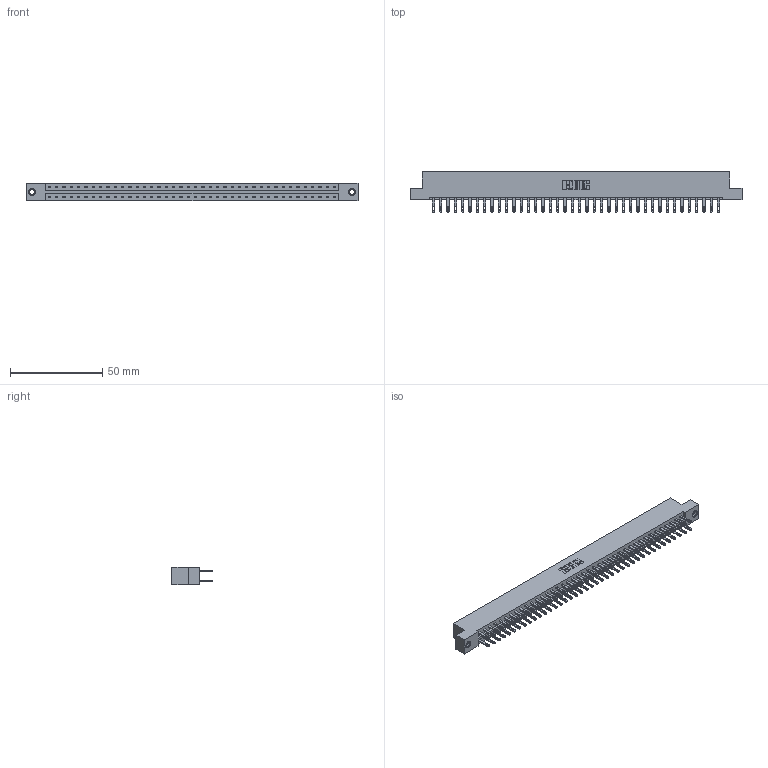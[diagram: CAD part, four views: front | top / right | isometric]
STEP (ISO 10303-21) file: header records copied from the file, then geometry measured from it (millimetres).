
FILE_DESCRIPTION (( 'STEP AP203' ), '1' );
FILE_NAME ('333-080-500-207.STEP', '2018-08-05T01:05:04', ( '' ), ( '' ), 'SwSTEP 2.0', 'SolidWorks 2016', '' );
FILE_SCHEMA (( 'CONFIG_CONTROL_DESIGN' ));
Length unit declared in the file: inch
Products named in the file (4): 333 Part_Flush - .156 Dia - TI; 345-292-001_345-293-100; 345-250-001_345-250-005-103; 333-080-500-207
Assembly tree (83 placements, depth 2):
  333-080-500-207
    333 Part_Flush - .156 Dia - TI
    345-292-001_345-293-100  x80
    345-250-001_345-250-005-103  x2
Bounding box: 180.04 x 21.85 x 9.4 mm (x, y, z)
Volume: 18592.8 mm3; surface area: 22874.3 mm2
Topology: 83 solids, 83 shells, 4014 faces, 12207 edges, 8130 vertices
Faces by surface type: plane 2502, cylinder 1496, cone 12, torus 4
Entity records: 27108 total; most frequent: CARTESIAN_POINT 4477, ORIENTED_EDGE 4406, DIRECTION 3861, EDGE_CURVE 2203, VECTOR 2051, LINE 2051, VERTEX_POINT 1464, AXIS2_PLACEMENT_3D 905
